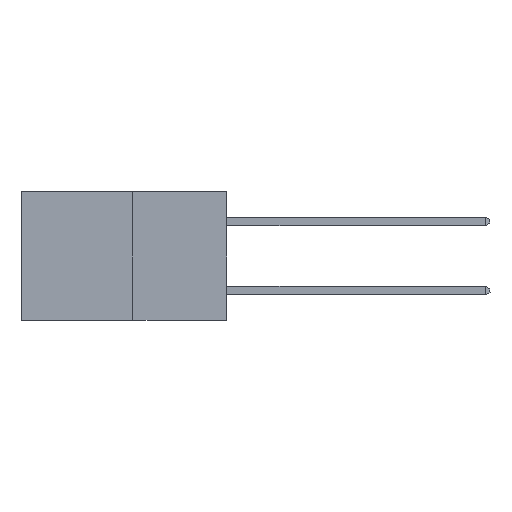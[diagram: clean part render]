
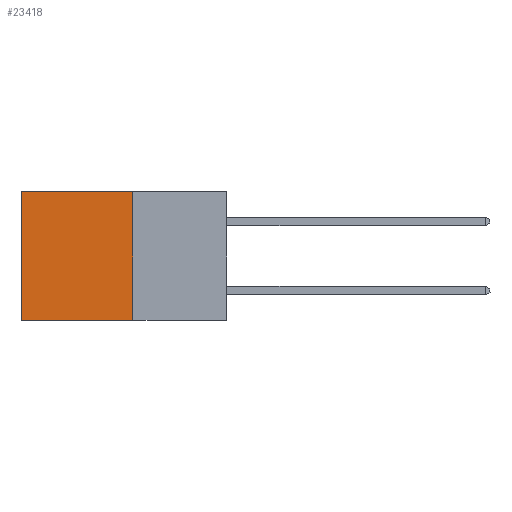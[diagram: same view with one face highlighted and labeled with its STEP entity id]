
A CAD part, left-side view. The second image highlights one B-rep face of the part: STEP entity #23418.
In plain terms, the highlighted planar face has unit normal (-1, 0, 0).
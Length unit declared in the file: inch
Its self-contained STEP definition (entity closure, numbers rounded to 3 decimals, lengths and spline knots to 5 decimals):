
#1234 = ORIENTED_EDGE ( 'NONE', *, *, #11698, .T. ) ;
#1891 = ORIENTED_EDGE ( 'NONE', *, *, #12598, .T. ) ;
#2691 = CARTESIAN_POINT ( 'NONE',  ( 0.277, 0.27, -0.37 ) ) ;
#2957 = CARTESIAN_POINT ( 'NONE',  ( 0.277, 0.27, -0.37 ) ) ;
#3273 = VECTOR ( 'NONE', #13537, 39.37008 ) ;
#4346 = VERTEX_POINT ( 'NONE', #7757 ) ;
#7510 = CARTESIAN_POINT ( 'NONE',  ( 0.277, 0.59, -0.37 ) ) ;
#7757 = CARTESIAN_POINT ( 'NONE',  ( 0.277, 0.27, -0.37 ) ) ;
#8307 = DIRECTION ( 'NONE',  ( 0., 0., -1. ) ) ;
#9661 = VERTEX_POINT ( 'NONE', #24747 ) ;
#10293 = VECTOR ( 'NONE', #26705, 39.37008 ) ;
#10720 = VERTEX_POINT ( 'NONE', #7510 ) ;
#11698 = EDGE_CURVE ( 'NONE', #15074, #10720, #29167, .T. ) ;
#12598 = EDGE_CURVE ( 'NONE', #9661, #15074, #29099, .T. ) ;
#13537 = DIRECTION ( 'NONE',  ( 0., 1., 0. ) ) ;
#13592 = DIRECTION ( 'NONE',  ( 1., 0., 0. ) ) ;
#15074 = VERTEX_POINT ( 'NONE', #17663 ) ;
#17458 = LINE ( 'NONE', #26796, #3273 ) ;
#17663 = CARTESIAN_POINT ( 'NONE',  ( 0.277, 0.59, 0. ) ) ;
#18895 = ORIENTED_EDGE ( 'NONE', *, *, #19149, .F. ) ;
#19149 = EDGE_CURVE ( 'NONE', #4346, #10720, #17458, .T. ) ;
#21141 = EDGE_CURVE ( 'NONE', #9661, #4346, #33215, .T. ) ;
#22981 = ORIENTED_EDGE ( 'NONE', *, *, #21141, .F. ) ;
#23218 = EDGE_LOOP ( 'NONE', ( #1234, #18895, #22981, #1891 ) ) ;
#23418 = ADVANCED_FACE ( 'NONE', ( #29697 ), #24348, .F. ) ;
#24348 = PLANE ( 'NONE',  #27927 ) ;
#24747 = CARTESIAN_POINT ( 'NONE',  ( 0.277, 0.27, 0. ) ) ;
#26705 = DIRECTION ( 'NONE',  ( 0., 0., -1. ) ) ;
#26796 = CARTESIAN_POINT ( 'NONE',  ( 0.277, 0.27, -0.37 ) ) ;
#27927 = AXIS2_PLACEMENT_3D ( 'NONE', #2957, #13592, #8307 ) ;
#28258 = VECTOR ( 'NONE', #31804, 39.37008 ) ;
#29099 = LINE ( 'NONE', #29118, #28258 ) ;
#29118 = CARTESIAN_POINT ( 'NONE',  ( 0.277, 0.27, 0. ) ) ;
#29167 = LINE ( 'NONE', #29931, #32210 ) ;
#29697 = FACE_OUTER_BOUND ( 'NONE', #23218, .T. ) ;
#29931 = CARTESIAN_POINT ( 'NONE',  ( 0.277, 0.59, -0.37 ) ) ;
#31804 = DIRECTION ( 'NONE',  ( 0., 1., 0. ) ) ;
#32210 = VECTOR ( 'NONE', #32607, 39.37008 ) ;
#32607 = DIRECTION ( 'NONE',  ( 0., 0., -1. ) ) ;
#33215 = LINE ( 'NONE', #2691, #10293 ) ;
